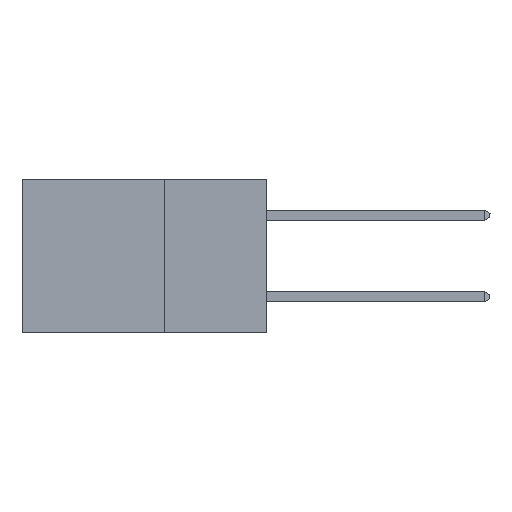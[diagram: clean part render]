
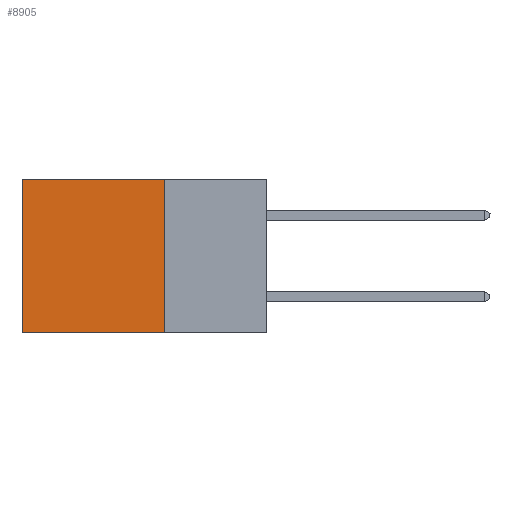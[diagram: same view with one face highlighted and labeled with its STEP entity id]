
A CAD part, left-side view. The second image highlights one B-rep face of the part: STEP entity #8905.
In plain terms, the highlighted planar face has unit normal (-1, 0, 0).
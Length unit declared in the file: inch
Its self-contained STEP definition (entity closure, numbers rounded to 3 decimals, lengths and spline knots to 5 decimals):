
#141 = LINE ( 'NONE', #12750, #14327 ) ;
#178 = CARTESIAN_POINT ( 'NONE',  ( 0.2875, 0.6, -0.375 ) ) ;
#517 = DIRECTION ( 'NONE',  ( 0., 0., -1. ) ) ;
#623 = CARTESIAN_POINT ( 'NONE',  ( 0.2875, 0.25, 0. ) ) ;
#721 = CARTESIAN_POINT ( 'NONE',  ( 0.2875, 0.6, 0. ) ) ;
#1088 = VECTOR ( 'NONE', #11994, 39.37008 ) ;
#1324 = DIRECTION ( 'NONE',  ( 1., 0., 0. ) ) ;
#2392 = VERTEX_POINT ( 'NONE', #623 ) ;
#2461 = PLANE ( 'NONE',  #6658 ) ;
#2592 = EDGE_CURVE ( 'NONE', #10714, #14563, #14716, .T. ) ;
#2679 = ORIENTED_EDGE ( 'NONE', *, *, #3207, .T. ) ;
#3003 = LINE ( 'NONE', #4071, #1088 ) ;
#3207 = EDGE_CURVE ( 'NONE', #14325, #14563, #5267, .T. ) ;
#4071 = CARTESIAN_POINT ( 'NONE',  ( 0.2875, 0.25, 0. ) ) ;
#4924 = ORIENTED_EDGE ( 'NONE', *, *, #2592, .F. ) ;
#5267 = LINE ( 'NONE', #14303, #8158 ) ;
#5842 = DIRECTION ( 'NONE',  ( 0., 0., -1. ) ) ;
#6658 = AXIS2_PLACEMENT_3D ( 'NONE', #12866, #1324, #5842 ) ;
#7052 = FACE_OUTER_BOUND ( 'NONE', #13816, .T. ) ;
#7498 = EDGE_CURVE ( 'NONE', #2392, #10714, #141, .T. ) ;
#7997 = DIRECTION ( 'NONE',  ( 0., 1., 0. ) ) ;
#8158 = VECTOR ( 'NONE', #517, 39.37008 ) ;
#8905 = ADVANCED_FACE ( 'NONE', ( #7052 ), #2461, .F. ) ;
#8969 = CARTESIAN_POINT ( 'NONE',  ( 0.2875, 0.25, -0.375 ) ) ;
#9338 = DIRECTION ( 'NONE',  ( 0., 0., -1. ) ) ;
#9351 = VECTOR ( 'NONE', #7997, 39.37008 ) ;
#10714 = VERTEX_POINT ( 'NONE', #12526 ) ;
#11994 = DIRECTION ( 'NONE',  ( 0., 1., 0. ) ) ;
#12526 = CARTESIAN_POINT ( 'NONE',  ( 0.2875, 0.25, -0.375 ) ) ;
#12750 = CARTESIAN_POINT ( 'NONE',  ( 0.2875, 0.25, -0.375 ) ) ;
#12866 = CARTESIAN_POINT ( 'NONE',  ( 0.2875, 0.25, -0.375 ) ) ;
#13311 = EDGE_CURVE ( 'NONE', #2392, #14325, #3003, .T. ) ;
#13353 = ORIENTED_EDGE ( 'NONE', *, *, #7498, .F. ) ;
#13816 = EDGE_LOOP ( 'NONE', ( #2679, #4924, #13353, #14855 ) ) ;
#14303 = CARTESIAN_POINT ( 'NONE',  ( 0.2875, 0.6, -0.375 ) ) ;
#14325 = VERTEX_POINT ( 'NONE', #721 ) ;
#14327 = VECTOR ( 'NONE', #9338, 39.37008 ) ;
#14563 = VERTEX_POINT ( 'NONE', #178 ) ;
#14716 = LINE ( 'NONE', #8969, #9351 ) ;
#14855 = ORIENTED_EDGE ( 'NONE', *, *, #13311, .T. ) ;
